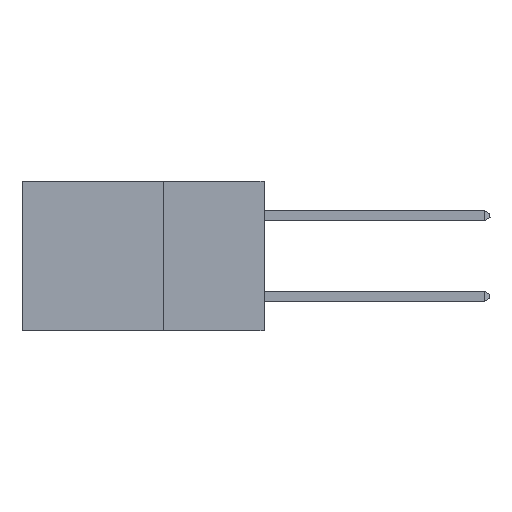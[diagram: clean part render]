
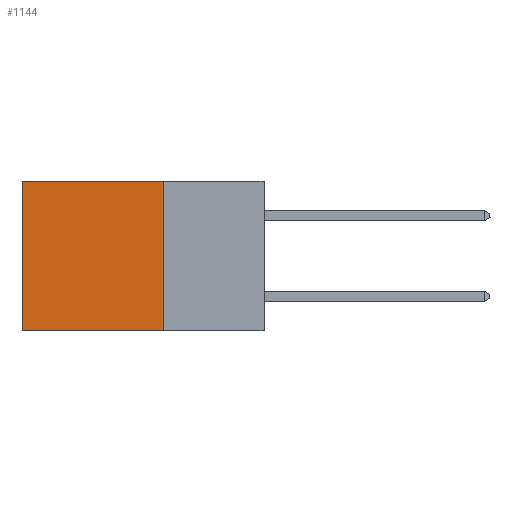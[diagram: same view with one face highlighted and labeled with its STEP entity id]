
A CAD part, left-side view. The second image highlights one B-rep face of the part: STEP entity #1144.
In plain terms, the highlighted planar face has unit normal (-1, 0, 0).
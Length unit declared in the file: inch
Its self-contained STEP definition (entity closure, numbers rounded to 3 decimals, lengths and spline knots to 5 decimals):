
#451 = CARTESIAN_POINT ( 'NONE',  ( 0.298, 0.25, 0. ) ) ;
#1144 = ADVANCED_FACE ( 'NONE', ( #11138 ), #9486, .F. ) ;
#2431 = VECTOR ( 'NONE', #5069, 39.37008 ) ;
#3026 = VERTEX_POINT ( 'NONE', #3193 ) ;
#3193 = CARTESIAN_POINT ( 'NONE',  ( 0.298, 0.25, -0.37 ) ) ;
#3238 = LINE ( 'NONE', #17514, #15466 ) ;
#4866 = VERTEX_POINT ( 'NONE', #12421 ) ;
#4933 = CARTESIAN_POINT ( 'NONE',  ( 0.298, 0.25, 0. ) ) ;
#4997 = LINE ( 'NONE', #5328, #2431 ) ;
#5027 = VERTEX_POINT ( 'NONE', #451 ) ;
#5069 = DIRECTION ( 'NONE',  ( 0., 0., -1. ) ) ;
#5328 = CARTESIAN_POINT ( 'NONE',  ( 0.298, 0.6, 0. ) ) ;
#5788 = EDGE_CURVE ( 'NONE', #4866, #15239, #4997, .T. ) ;
#6073 = VECTOR ( 'NONE', #24323, 39.37008 ) ;
#6796 = DIRECTION ( 'NONE',  ( 0., 1., 0. ) ) ;
#8762 = EDGE_CURVE ( 'NONE', #3026, #15239, #13784, .T. ) ;
#9486 = PLANE ( 'NONE',  #25625 ) ;
#11138 = FACE_OUTER_BOUND ( 'NONE', #26195, .T. ) ;
#11220 = DIRECTION ( 'NONE',  ( 0., 0., -1. ) ) ;
#12421 = CARTESIAN_POINT ( 'NONE',  ( 0.298, 0.6, 0. ) ) ;
#13289 = VECTOR ( 'NONE', #6796, 39.37008 ) ;
#13602 = LINE ( 'NONE', #4933, #13289 ) ;
#13784 = LINE ( 'NONE', #26223, #6073 ) ;
#13801 = EDGE_CURVE ( 'NONE', #5027, #3026, #3238, .T. ) ;
#13893 = ORIENTED_EDGE ( 'NONE', *, *, #5788, .T. ) ;
#13934 = ORIENTED_EDGE ( 'NONE', *, *, #8762, .F. ) ;
#14775 = ORIENTED_EDGE ( 'NONE', *, *, #13801, .F. ) ;
#15239 = VERTEX_POINT ( 'NONE', #24774 ) ;
#15466 = VECTOR ( 'NONE', #19852, 39.37008 ) ;
#15626 = DIRECTION ( 'NONE',  ( 1., 0., 0. ) ) ;
#17514 = CARTESIAN_POINT ( 'NONE',  ( 0.298, 0.25, 0. ) ) ;
#19852 = DIRECTION ( 'NONE',  ( 0., 0., -1. ) ) ;
#21880 = ORIENTED_EDGE ( 'NONE', *, *, #22403, .T. ) ;
#22403 = EDGE_CURVE ( 'NONE', #5027, #4866, #13602, .T. ) ;
#24323 = DIRECTION ( 'NONE',  ( 0., 1., 0. ) ) ;
#24774 = CARTESIAN_POINT ( 'NONE',  ( 0.298, 0.6, -0.37 ) ) ;
#25625 = AXIS2_PLACEMENT_3D ( 'NONE', #25742, #15626, #11220 ) ;
#25742 = CARTESIAN_POINT ( 'NONE',  ( 0.298, 0.25, 0. ) ) ;
#26195 = EDGE_LOOP ( 'NONE', ( #13893, #13934, #14775, #21880 ) ) ;
#26223 = CARTESIAN_POINT ( 'NONE',  ( 0.298, 0.25, -0.37 ) ) ;
